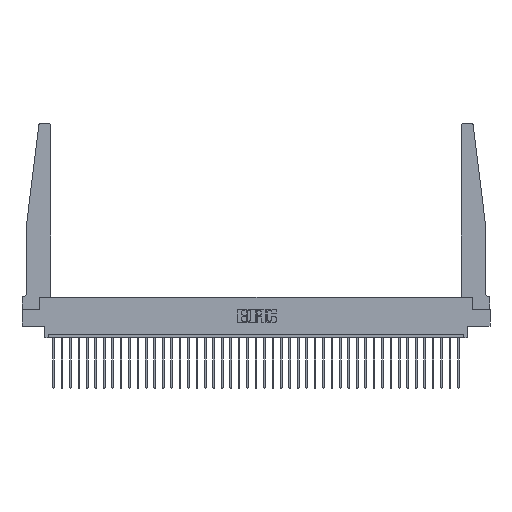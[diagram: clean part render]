
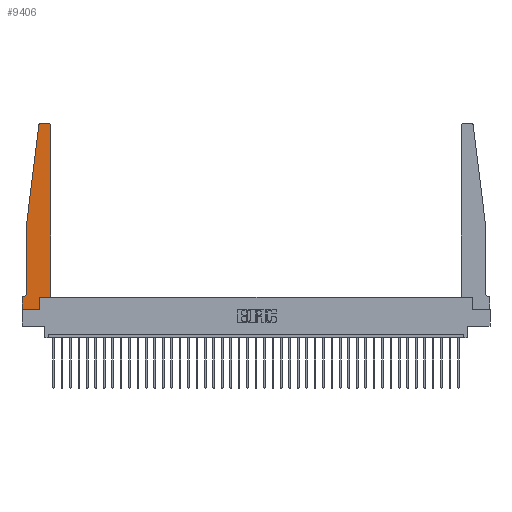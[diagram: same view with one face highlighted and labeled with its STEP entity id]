
A CAD part, top view. The second image highlights one B-rep face of the part: STEP entity #9406.
In plain terms, the highlighted planar face has unit normal (0, 0, 1).
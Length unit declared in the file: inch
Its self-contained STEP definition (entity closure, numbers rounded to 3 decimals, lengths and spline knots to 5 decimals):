
#356 = EDGE_CURVE ( 'NONE', #18129, #6630, #20788, .T. ) ;
#486 = VERTEX_POINT ( 'NONE', #29691 ) ;
#533 = PLANE ( 'NONE',  #15359 ) ;
#583 = CARTESIAN_POINT ( 'NONE',  ( 0.2605, 0.18, 0.37 ) ) ;
#737 = LINE ( 'NONE', #23842, #26084 ) ;
#958 = VERTEX_POINT ( 'NONE', #22648 ) ;
#1522 = EDGE_CURVE ( 'NONE', #10134, #958, #18701, .T. ) ;
#1868 = DIRECTION ( 'NONE',  ( 1., 0., 0. ) ) ;
#2079 = AXIS2_PLACEMENT_3D ( 'NONE', #9209, #14233, #14355 ) ;
#2139 = VERTEX_POINT ( 'NONE', #21798 ) ;
#2576 = CARTESIAN_POINT ( 'NONE',  ( 0., 0., 0.37 ) ) ;
#2598 = ORIENTED_EDGE ( 'NONE', *, *, #28831, .T. ) ;
#2703 = ORIENTED_EDGE ( 'NONE', *, *, #16592, .T. ) ;
#2823 = ORIENTED_EDGE ( 'NONE', *, *, #13819, .T. ) ;
#3411 = CARTESIAN_POINT ( 'NONE',  ( 0.425, 0.18, 0.37 ) ) ;
#3512 = VECTOR ( 'NONE', #25664, 39.37008 ) ;
#5331 = VECTOR ( 'NONE', #6953, 39.37008 ) ;
#5816 = CARTESIAN_POINT ( 'NONE',  ( 0.395, 2.72, 0.37 ) ) ;
#5854 = VERTEX_POINT ( 'NONE', #22595 ) ;
#6209 = CARTESIAN_POINT ( 'NONE',  ( 0.425, 0.18, 0.37 ) ) ;
#6343 = LINE ( 'NONE', #3411, #7621 ) ;
#6630 = VERTEX_POINT ( 'NONE', #6209 ) ;
#6950 = CARTESIAN_POINT ( 'NONE',  ( 0., 0., 0.37 ) ) ;
#6953 = DIRECTION ( 'NONE',  ( 0., -1., 0. ) ) ;
#7621 = VECTOR ( 'NONE', #27231, 39.37008 ) ;
#7813 = ORIENTED_EDGE ( 'NONE', *, *, #14536, .T. ) ;
#7852 = EDGE_CURVE ( 'NONE', #13207, #17301, #22263, .T. ) ;
#8858 = ORIENTED_EDGE ( 'NONE', *, *, #33970, .T. ) ;
#9209 = CARTESIAN_POINT ( 'NONE',  ( 0.27653, 2.72, 0.37 ) ) ;
#9406 = ADVANCED_FACE ( 'NONE', ( #26735 ), #533, .T. ) ;
#9810 = EDGE_CURVE ( 'NONE', #6630, #5854, #6343, .T. ) ;
#10132 = AXIS2_PLACEMENT_3D ( 'NONE', #11928, #27697, #14249 ) ;
#10134 = VERTEX_POINT ( 'NONE', #29887 ) ;
#11564 = DIRECTION ( 'NONE',  ( 0., 0., 1. ) ) ;
#11928 = CARTESIAN_POINT ( 'NONE',  ( 0.015, 0.2375, 0.37 ) ) ;
#12252 = CARTESIAN_POINT ( 'NONE',  ( 0., 0., 0.37 ) ) ;
#12723 = AXIS2_PLACEMENT_3D ( 'NONE', #5816, #11564, #17023 ) ;
#12994 = VERTEX_POINT ( 'NONE', #19676 ) ;
#13207 = VERTEX_POINT ( 'NONE', #24452 ) ;
#13737 = VECTOR ( 'NONE', #1868, 39.37008 ) ;
#13819 = EDGE_CURVE ( 'NONE', #28935, #12994, #29457, .T. ) ;
#14233 = DIRECTION ( 'NONE',  ( 0., 0., 1. ) ) ;
#14249 = DIRECTION ( 'NONE',  ( -1., 0., 0. ) ) ;
#14355 = DIRECTION ( 'NONE',  ( 1., 0., 0. ) ) ;
#14536 = EDGE_CURVE ( 'NONE', #16594, #13207, #737, .T. ) ;
#14875 = ORIENTED_EDGE ( 'NONE', *, *, #7852, .T. ) ;
#15359 = AXIS2_PLACEMENT_3D ( 'NONE', #29569, #16359, #24346 ) ;
#15481 = VECTOR ( 'NONE', #27959, 39.37008 ) ;
#15742 = CARTESIAN_POINT ( 'NONE',  ( 0.25, 2.75, 0.37 ) ) ;
#16359 = DIRECTION ( 'NONE',  ( 0., 0., 1. ) ) ;
#16536 = ORIENTED_EDGE ( 'NONE', *, *, #356, .T. ) ;
#16592 = EDGE_CURVE ( 'NONE', #958, #486, #31716, .T. ) ;
#16594 = VERTEX_POINT ( 'NONE', #22571 ) ;
#17023 = DIRECTION ( 'NONE',  ( 1., 0., 0. ) ) ;
#17301 = VERTEX_POINT ( 'NONE', #2576 ) ;
#17308 = VECTOR ( 'NONE', #28221, 39.37008 ) ;
#17655 = CARTESIAN_POINT ( 'NONE',  ( 0.2605, 0.18, 0.37 ) ) ;
#18129 = VERTEX_POINT ( 'NONE', #583 ) ;
#18376 = VECTOR ( 'NONE', #19336, 39.37008 ) ;
#18701 = LINE ( 'NONE', #15742, #30733 ) ;
#18751 = LINE ( 'NONE', #29993, #18376 ) ;
#19336 = DIRECTION ( 'NONE',  ( -0.122, -0.992, 0. ) ) ;
#19676 = CARTESIAN_POINT ( 'NONE',  ( 0.065, 0.2375, 0.37 ) ) ;
#20057 = ORIENTED_EDGE ( 'NONE', *, *, #27569, .T. ) ;
#20677 = ORIENTED_EDGE ( 'NONE', *, *, #9810, .T. ) ;
#20788 = LINE ( 'NONE', #25368, #13737 ) ;
#21798 = CARTESIAN_POINT ( 'NONE',  ( 0.2605, 0., 0.37 ) ) ;
#22263 = LINE ( 'NONE', #12252, #3512 ) ;
#22571 = CARTESIAN_POINT ( 'NONE',  ( 0.015, 0.1875, 0.37 ) ) ;
#22595 = CARTESIAN_POINT ( 'NONE',  ( 0.425, 2.72, 0.37 ) ) ;
#22648 = CARTESIAN_POINT ( 'NONE',  ( 0.27653, 2.75, 0.37 ) ) ;
#23198 = CIRCLE ( 'NONE', #10132, 0.05 ) ;
#23220 = CIRCLE ( 'NONE', #12723, 0.03 ) ;
#23251 = EDGE_CURVE ( 'NONE', #2139, #18129, #27087, .T. ) ;
#23413 = ORIENTED_EDGE ( 'NONE', *, *, #23251, .T. ) ;
#23647 = ORIENTED_EDGE ( 'NONE', *, *, #1522, .T. ) ;
#23842 = CARTESIAN_POINT ( 'NONE',  ( 0.065, 0.1875, 0.37 ) ) ;
#24171 = EDGE_CURVE ( 'NONE', #486, #28935, #18751, .T. ) ;
#24346 = DIRECTION ( 'NONE',  ( 1., 0., 0. ) ) ;
#24452 = CARTESIAN_POINT ( 'NONE',  ( 0., 0.1875, 0.37 ) ) ;
#25368 = CARTESIAN_POINT ( 'NONE',  ( 0.425, 0.18, 0.37 ) ) ;
#25664 = DIRECTION ( 'NONE',  ( 0., -1., 0. ) ) ;
#25918 = DIRECTION ( 'NONE',  ( -1., 0., 0. ) ) ;
#26084 = VECTOR ( 'NONE', #34271, 39.37008 ) ;
#26735 = FACE_OUTER_BOUND ( 'NONE', #28944, .T. ) ;
#27087 = LINE ( 'NONE', #17655, #15481 ) ;
#27231 = DIRECTION ( 'NONE',  ( 0., 1., 0. ) ) ;
#27569 = EDGE_CURVE ( 'NONE', #5854, #10134, #23220, .T. ) ;
#27697 = DIRECTION ( 'NONE',  ( 0., 0., -1. ) ) ;
#27959 = DIRECTION ( 'NONE',  ( 0., 1., 0. ) ) ;
#28012 = ORIENTED_EDGE ( 'NONE', *, *, #24171, .T. ) ;
#28112 = CARTESIAN_POINT ( 'NONE',  ( 0.065, 1.25, 0.37 ) ) ;
#28221 = DIRECTION ( 'NONE',  ( 1., 0., 0. ) ) ;
#28831 = EDGE_CURVE ( 'NONE', #17301, #2139, #29750, .T. ) ;
#28935 = VERTEX_POINT ( 'NONE', #30038 ) ;
#28944 = EDGE_LOOP ( 'NONE', ( #23647, #2703, #28012, #2823, #8858, #7813, #14875, #2598, #23413, #16536, #20677, #20057 ) ) ;
#29457 = LINE ( 'NONE', #28112, #5331 ) ;
#29569 = CARTESIAN_POINT ( 'NONE',  ( 0., 0.1875, 0.37 ) ) ;
#29691 = CARTESIAN_POINT ( 'NONE',  ( 0.24675, 2.72367, 0.37 ) ) ;
#29750 = LINE ( 'NONE', #6950, #17308 ) ;
#29887 = CARTESIAN_POINT ( 'NONE',  ( 0.395, 2.75, 0.37 ) ) ;
#29993 = CARTESIAN_POINT ( 'NONE',  ( 0.065, 1.25, 0.37 ) ) ;
#30038 = CARTESIAN_POINT ( 'NONE',  ( 0.065, 1.25, 0.37 ) ) ;
#30733 = VECTOR ( 'NONE', #25918, 39.37008 ) ;
#31716 = CIRCLE ( 'NONE', #2079, 0.03 ) ;
#33970 = EDGE_CURVE ( 'NONE', #12994, #16594, #23198, .T. ) ;
#34271 = DIRECTION ( 'NONE',  ( -1., 0., 0. ) ) ;
